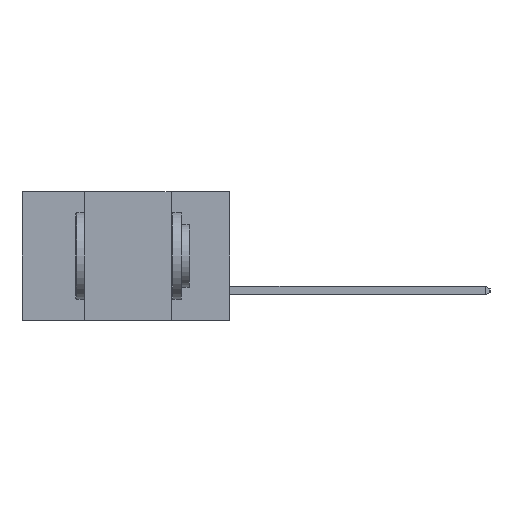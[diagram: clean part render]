
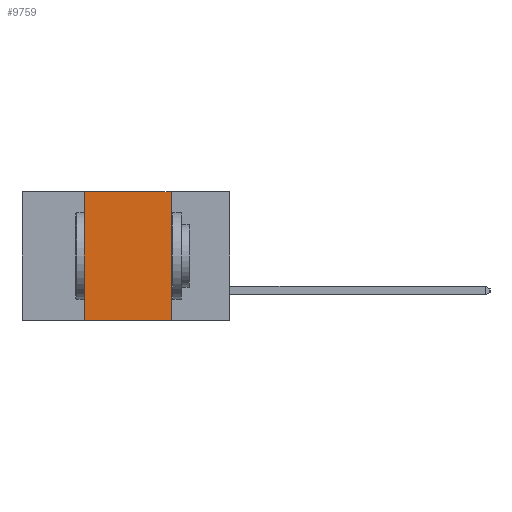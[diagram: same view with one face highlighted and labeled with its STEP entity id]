
A CAD part, left-side view. The second image highlights one B-rep face of the part: STEP entity #9759.
In plain terms, the highlighted planar face has unit normal (-1, 0, 0).
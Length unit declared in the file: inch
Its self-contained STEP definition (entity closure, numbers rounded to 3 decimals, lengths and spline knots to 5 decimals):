
#393 = EDGE_CURVE ( 'NONE', #12246, #5230, #6413, .T. ) ;
#394 = LINE ( 'NONE', #11381, #5475 ) ;
#469 = CARTESIAN_POINT ( 'NONE',  ( 0., 0.42, 0. ) ) ;
#851 = VERTEX_POINT ( 'NONE', #469 ) ;
#882 = CARTESIAN_POINT ( 'NONE',  ( 0., 0.6, -0.37 ) ) ;
#1127 = VECTOR ( 'NONE', #4582, 39.37008 ) ;
#1746 = VERTEX_POINT ( 'NONE', #7326 ) ;
#1898 = LINE ( 'NONE', #882, #9237 ) ;
#1903 = VECTOR ( 'NONE', #7469, 39.37008 ) ;
#1937 = DIRECTION ( 'NONE',  ( 0., 0., -1. ) ) ;
#1982 = DIRECTION ( 'NONE',  ( 0., -1., 0. ) ) ;
#1989 = DIRECTION ( 'NONE',  ( 1., 0., 0. ) ) ;
#2006 = CARTESIAN_POINT ( 'NONE',  ( 0., 0.6, 0. ) ) ;
#2241 = PLANE ( 'NONE',  #10599 ) ;
#2330 = CARTESIAN_POINT ( 'NONE',  ( 0., 0.17, -0.37 ) ) ;
#4031 = EDGE_CURVE ( 'NONE', #851, #12246, #7068, .T. ) ;
#4582 = DIRECTION ( 'NONE',  ( 0., 0., -1. ) ) ;
#4914 = CARTESIAN_POINT ( 'NONE',  ( 0., 0.17, 0. ) ) ;
#5230 = VERTEX_POINT ( 'NONE', #2330 ) ;
#5475 = VECTOR ( 'NONE', #10063, 39.37008 ) ;
#6299 = EDGE_LOOP ( 'NONE', ( #6966, #6688, #8846, #6378 ) ) ;
#6378 = ORIENTED_EDGE ( 'NONE', *, *, #11184, .T. ) ;
#6413 = LINE ( 'NONE', #6513, #1127 ) ;
#6513 = CARTESIAN_POINT ( 'NONE',  ( 0., 0.17, -0.37 ) ) ;
#6688 = ORIENTED_EDGE ( 'NONE', *, *, #4031, .F. ) ;
#6966 = ORIENTED_EDGE ( 'NONE', *, *, #393, .F. ) ;
#7068 = LINE ( 'NONE', #7472, #1903 ) ;
#7326 = CARTESIAN_POINT ( 'NONE',  ( 0., 0.42, -0.37 ) ) ;
#7469 = DIRECTION ( 'NONE',  ( 0., -1., 0. ) ) ;
#7472 = CARTESIAN_POINT ( 'NONE',  ( 0., 0.6, 0. ) ) ;
#8555 = FACE_OUTER_BOUND ( 'NONE', #6299, .T. ) ;
#8846 = ORIENTED_EDGE ( 'NONE', *, *, #10233, .F. ) ;
#9237 = VECTOR ( 'NONE', #1982, 39.37008 ) ;
#9759 = ADVANCED_FACE ( 'NONE', ( #8555 ), #2241, .F. ) ;
#10063 = DIRECTION ( 'NONE',  ( 0., 0., 1. ) ) ;
#10233 = EDGE_CURVE ( 'NONE', #1746, #851, #394, .T. ) ;
#10599 = AXIS2_PLACEMENT_3D ( 'NONE', #2006, #1989, #1937 ) ;
#11184 = EDGE_CURVE ( 'NONE', #1746, #5230, #1898, .T. ) ;
#11381 = CARTESIAN_POINT ( 'NONE',  ( 0., 0.42, -0.37 ) ) ;
#12246 = VERTEX_POINT ( 'NONE', #4914 ) ;
